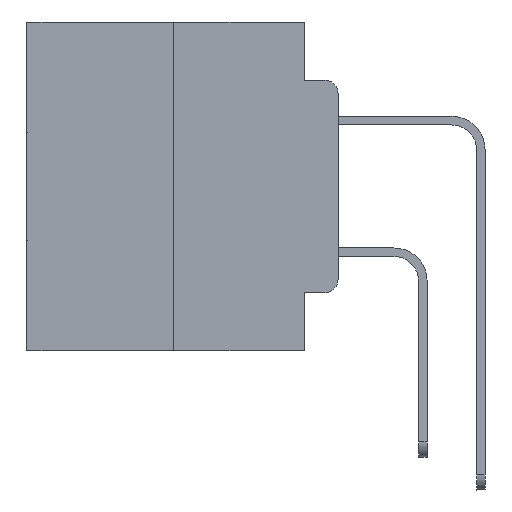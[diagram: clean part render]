
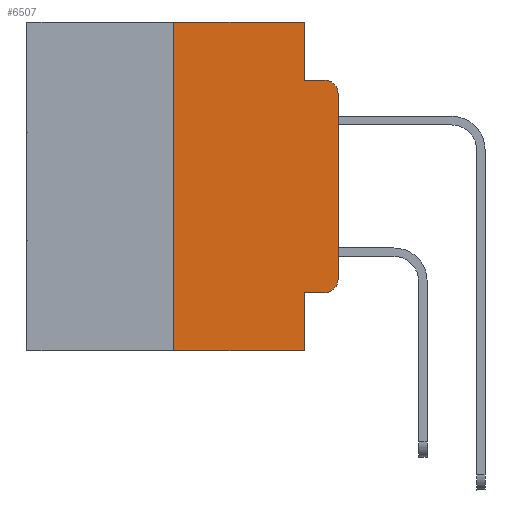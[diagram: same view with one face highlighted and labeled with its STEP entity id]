
A CAD part, left-side view. The second image highlights one B-rep face of the part: STEP entity #6507.
In plain terms, the highlighted planar face has unit normal (-1, 0, 0).
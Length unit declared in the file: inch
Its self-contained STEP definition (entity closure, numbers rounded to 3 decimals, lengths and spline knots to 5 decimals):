
#25 = CARTESIAN_POINT ( 'NONE',  ( 0., 0.02, -0.4115 ) ) ;
#59 = VERTEX_POINT ( 'NONE', #11645 ) ;
#105 = DIRECTION ( 'NONE',  ( 0., -1., 0. ) ) ;
#167 = CARTESIAN_POINT ( 'NONE',  ( 0., 0.473, 0. ) ) ;
#201 = DIRECTION ( 'NONE',  ( 0., 0., -1. ) ) ;
#354 = EDGE_CURVE ( 'NONE', #12610, #2408, #14272, .T. ) ;
#778 = CARTESIAN_POINT ( 'NONE',  ( 0., 0., -0.3915 ) ) ;
#1193 = VECTOR ( 'NONE', #201, 39.37008 ) ;
#1309 = ORIENTED_EDGE ( 'NONE', *, *, #19241, .T. ) ;
#1973 = ORIENTED_EDGE ( 'NONE', *, *, #26651, .F. ) ;
#2108 = VERTEX_POINT ( 'NONE', #4242 ) ;
#2346 = CARTESIAN_POINT ( 'NONE',  ( 0., 0.051, -0.5 ) ) ;
#2408 = VERTEX_POINT ( 'NONE', #6780 ) ;
#2690 = LINE ( 'NONE', #15339, #20106 ) ;
#2844 = VECTOR ( 'NONE', #12892, 39.37008 ) ;
#3418 = EDGE_CURVE ( 'NONE', #24993, #2408, #16705, .T. ) ;
#3427 = CARTESIAN_POINT ( 'NONE',  ( 0., 0.473, 0. ) ) ;
#4242 = CARTESIAN_POINT ( 'NONE',  ( 0., 0.25, -0.5 ) ) ;
#4929 = EDGE_CURVE ( 'NONE', #10775, #24993, #5250, .T. ) ;
#5250 = LINE ( 'NONE', #26852, #5982 ) ;
#5482 = CARTESIAN_POINT ( 'NONE',  ( 0., 0.051, 0. ) ) ;
#5710 = DIRECTION ( 'NONE',  ( 1., 0., 0. ) ) ;
#5982 = VECTOR ( 'NONE', #13487, 39.37008 ) ;
#6214 = CARTESIAN_POINT ( 'NONE',  ( 0., 0.02, -0.3915 ) ) ;
#6507 = ADVANCED_FACE ( 'NONE', ( #24953 ), #10243, .F. ) ;
#6780 = CARTESIAN_POINT ( 'NONE',  ( 0., 0.02, -0.0885 ) ) ;
#6876 = EDGE_CURVE ( 'NONE', #2108, #16994, #25624, .T. ) ;
#7569 = LINE ( 'NONE', #5482, #18927 ) ;
#7670 = VECTOR ( 'NONE', #105, 39.37008 ) ;
#8543 = DIRECTION ( 'NONE',  ( 0., 0., -1. ) ) ;
#9137 = VECTOR ( 'NONE', #11573, 39.37008 ) ;
#9184 = VERTEX_POINT ( 'NONE', #14853 ) ;
#10243 = PLANE ( 'NONE',  #26743 ) ;
#10775 = VERTEX_POINT ( 'NONE', #778 ) ;
#11188 = CARTESIAN_POINT ( 'NONE',  ( 0., 0.051, -0.0885 ) ) ;
#11377 = DIRECTION ( 'NONE',  ( 0., 0., 1. ) ) ;
#11573 = DIRECTION ( 'NONE',  ( 0., -1., 0. ) ) ;
#11645 = CARTESIAN_POINT ( 'NONE',  ( 0., 0.25, 0. ) ) ;
#12390 = CIRCLE ( 'NONE', #12773, 0.02 ) ;
#12610 = VERTEX_POINT ( 'NONE', #27212 ) ;
#12773 = AXIS2_PLACEMENT_3D ( 'NONE', #6214, #22058, #8543 ) ;
#12892 = DIRECTION ( 'NONE',  ( 0., -1., 0. ) ) ;
#13487 = DIRECTION ( 'NONE',  ( 0., 0., 1. ) ) ;
#13781 = CARTESIAN_POINT ( 'NONE',  ( 0., 0.473, -0.5 ) ) ;
#14029 = DIRECTION ( 'NONE',  ( -1., 0., 0. ) ) ;
#14272 = LINE ( 'NONE', #11188, #2844 ) ;
#14678 = CARTESIAN_POINT ( 'NONE',  ( 0., 0., -0.1085 ) ) ;
#14853 = CARTESIAN_POINT ( 'NONE',  ( 0., 0.051, -0.4115 ) ) ;
#15208 = ORIENTED_EDGE ( 'NONE', *, *, #22211, .T. ) ;
#15339 = CARTESIAN_POINT ( 'NONE',  ( 0., 0.051, -0.4115 ) ) ;
#16705 = CIRCLE ( 'NONE', #18905, 0.02 ) ;
#16726 = DIRECTION ( 'NONE',  ( 0., 0., -1. ) ) ;
#16994 = VERTEX_POINT ( 'NONE', #2346 ) ;
#17605 = DIRECTION ( 'NONE',  ( 0., -1., 0. ) ) ;
#18087 = CARTESIAN_POINT ( 'NONE',  ( 0., 0.25, 0. ) ) ;
#18905 = AXIS2_PLACEMENT_3D ( 'NONE', #27377, #14029, #29025 ) ;
#18927 = VECTOR ( 'NONE', #16726, 39.37008 ) ;
#19241 = EDGE_CURVE ( 'NONE', #21794, #10775, #12390, .T. ) ;
#20066 = ORIENTED_EDGE ( 'NONE', *, *, #22419, .F. ) ;
#20106 = VECTOR ( 'NONE', #17605, 39.37008 ) ;
#20117 = CARTESIAN_POINT ( 'NONE',  ( 0., 0.051, 0. ) ) ;
#20333 = ORIENTED_EDGE ( 'NONE', *, *, #4929, .T. ) ;
#20793 = ORIENTED_EDGE ( 'NONE', *, *, #6876, .T. ) ;
#21134 = LINE ( 'NONE', #167, #9137 ) ;
#21561 = DIRECTION ( 'NONE',  ( 0., 0., -1. ) ) ;
#21794 = VERTEX_POINT ( 'NONE', #25 ) ;
#21931 = LINE ( 'NONE', #18087, #27100 ) ;
#22058 = DIRECTION ( 'NONE',  ( -1., 0., 0. ) ) ;
#22129 = ORIENTED_EDGE ( 'NONE', *, *, #354, .F. ) ;
#22211 = EDGE_CURVE ( 'NONE', #9184, #21794, #2690, .T. ) ;
#22419 = EDGE_CURVE ( 'NONE', #59, #22908, #21134, .T. ) ;
#22797 = CARTESIAN_POINT ( 'NONE',  ( 0., 0.051, 0. ) ) ;
#22908 = VERTEX_POINT ( 'NONE', #20117 ) ;
#23687 = EDGE_CURVE ( 'NONE', #9184, #16994, #25922, .T. ) ;
#24212 = ORIENTED_EDGE ( 'NONE', *, *, #28117, .F. ) ;
#24292 = ORIENTED_EDGE ( 'NONE', *, *, #23687, .F. ) ;
#24524 = ORIENTED_EDGE ( 'NONE', *, *, #3418, .T. ) ;
#24806 = EDGE_LOOP ( 'NONE', ( #20333, #24524, #22129, #24212, #20066, #1973, #20793, #24292, #15208, #1309 ) ) ;
#24953 = FACE_OUTER_BOUND ( 'NONE', #24806, .T. ) ;
#24993 = VERTEX_POINT ( 'NONE', #14678 ) ;
#25624 = LINE ( 'NONE', #13781, #7670 ) ;
#25922 = LINE ( 'NONE', #22797, #1193 ) ;
#26651 = EDGE_CURVE ( 'NONE', #2108, #59, #21931, .T. ) ;
#26743 = AXIS2_PLACEMENT_3D ( 'NONE', #3427, #5710, #21561 ) ;
#26852 = CARTESIAN_POINT ( 'NONE',  ( 0., 0., 0. ) ) ;
#27100 = VECTOR ( 'NONE', #11377, 39.37008 ) ;
#27212 = CARTESIAN_POINT ( 'NONE',  ( 0., 0.051, -0.0885 ) ) ;
#27377 = CARTESIAN_POINT ( 'NONE',  ( 0., 0.02, -0.1085 ) ) ;
#28117 = EDGE_CURVE ( 'NONE', #22908, #12610, #7569, .T. ) ;
#29025 = DIRECTION ( 'NONE',  ( 0., 0., -1. ) ) ;
